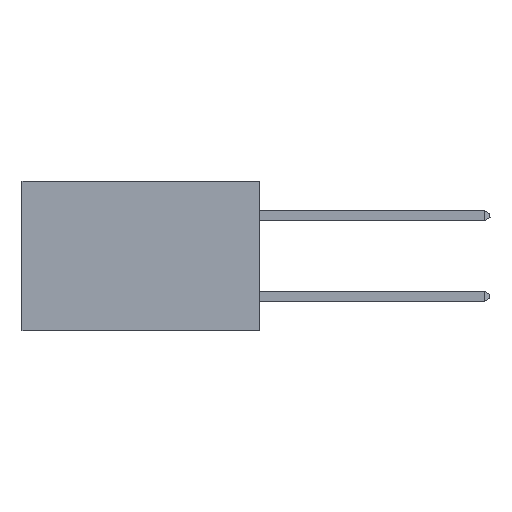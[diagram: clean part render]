
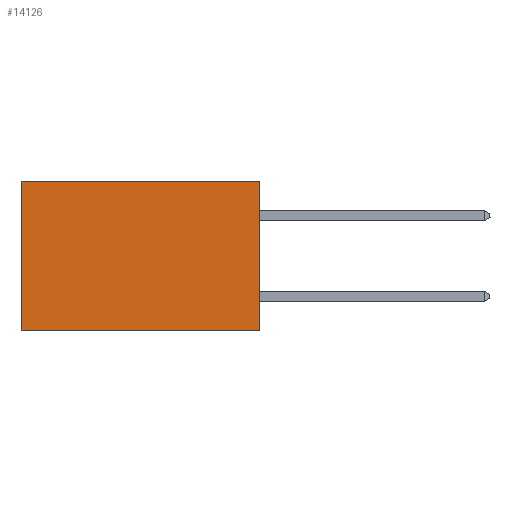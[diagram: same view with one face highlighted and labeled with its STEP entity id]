
A CAD part, left-side view. The second image highlights one B-rep face of the part: STEP entity #14126.
In plain terms, the highlighted planar face has unit normal (-1, 0, 0).
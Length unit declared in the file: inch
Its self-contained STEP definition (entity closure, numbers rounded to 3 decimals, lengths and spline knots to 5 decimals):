
#1356 = LINE ( 'NONE', #11689, #10251 ) ;
#1492 = VECTOR ( 'NONE', #4384, 39.37008 ) ;
#1586 = EDGE_CURVE ( 'NONE', #3560, #12790, #1356, .T. ) ;
#1669 = VERTEX_POINT ( 'NONE', #8788 ) ;
#3164 = CARTESIAN_POINT ( 'NONE',  ( 0.277, 0., -0.37 ) ) ;
#3560 = VERTEX_POINT ( 'NONE', #5843 ) ;
#4367 = VECTOR ( 'NONE', #8114, 39.37008 ) ;
#4384 = DIRECTION ( 'NONE',  ( 0., 1., 0. ) ) ;
#4438 = ORIENTED_EDGE ( 'NONE', *, *, #16673, .F. ) ;
#4984 = DIRECTION ( 'NONE',  ( 1., 0., 0. ) ) ;
#5843 = CARTESIAN_POINT ( 'NONE',  ( 0.277, 0., -0.37 ) ) ;
#6131 = ORIENTED_EDGE ( 'NONE', *, *, #10917, .T. ) ;
#6898 = ORIENTED_EDGE ( 'NONE', *, *, #10341, .T. ) ;
#8114 = DIRECTION ( 'NONE',  ( 0., 0., -1. ) ) ;
#8788 = CARTESIAN_POINT ( 'NONE',  ( 0.277, 0.59, 0. ) ) ;
#9607 = CARTESIAN_POINT ( 'NONE',  ( 0.277, 0., -0.37 ) ) ;
#10251 = VECTOR ( 'NONE', #15551, 39.37008 ) ;
#10341 = EDGE_CURVE ( 'NONE', #1669, #12790, #13700, .T. ) ;
#10917 = EDGE_CURVE ( 'NONE', #14231, #1669, #20092, .T. ) ;
#11689 = CARTESIAN_POINT ( 'NONE',  ( 0.277, 0., -0.37 ) ) ;
#11692 = CARTESIAN_POINT ( 'NONE',  ( 0.277, 0.59, -0.37 ) ) ;
#12201 = ORIENTED_EDGE ( 'NONE', *, *, #1586, .F. ) ;
#12790 = VERTEX_POINT ( 'NONE', #22080 ) ;
#12924 = EDGE_LOOP ( 'NONE', ( #6898, #12201, #4438, #6131 ) ) ;
#13131 = CARTESIAN_POINT ( 'NONE',  ( 0.277, 0., 0. ) ) ;
#13655 = LINE ( 'NONE', #9607, #19282 ) ;
#13700 = LINE ( 'NONE', #11692, #4367 ) ;
#13721 = PLANE ( 'NONE',  #16993 ) ;
#14126 = ADVANCED_FACE ( 'NONE', ( #14882 ), #13721, .F. ) ;
#14231 = VERTEX_POINT ( 'NONE', #20819 ) ;
#14882 = FACE_OUTER_BOUND ( 'NONE', #12924, .T. ) ;
#15551 = DIRECTION ( 'NONE',  ( 0., 1., 0. ) ) ;
#16673 = EDGE_CURVE ( 'NONE', #14231, #3560, #13655, .T. ) ;
#16993 = AXIS2_PLACEMENT_3D ( 'NONE', #3164, #4984, #17218 ) ;
#17218 = DIRECTION ( 'NONE',  ( 0., 0., -1. ) ) ;
#19282 = VECTOR ( 'NONE', #21654, 39.37008 ) ;
#20092 = LINE ( 'NONE', #13131, #1492 ) ;
#20819 = CARTESIAN_POINT ( 'NONE',  ( 0.277, 0., 0. ) ) ;
#21654 = DIRECTION ( 'NONE',  ( 0., 0., -1. ) ) ;
#22080 = CARTESIAN_POINT ( 'NONE',  ( 0.277, 0.59, -0.37 ) ) ;
